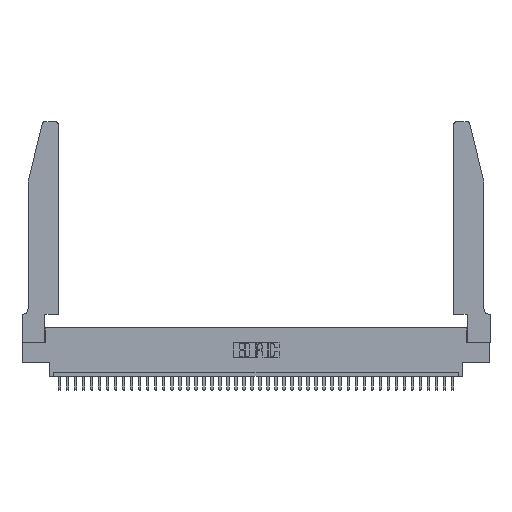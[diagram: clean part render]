
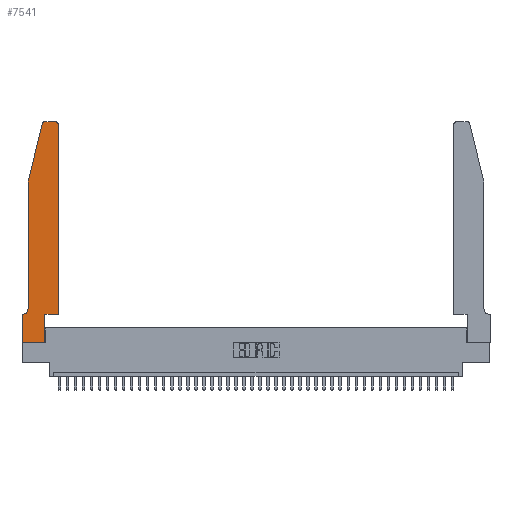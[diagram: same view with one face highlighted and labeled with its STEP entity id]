
A CAD part, top view. The second image highlights one B-rep face of the part: STEP entity #7541.
In plain terms, the highlighted planar face has unit normal (0, 0, 1).
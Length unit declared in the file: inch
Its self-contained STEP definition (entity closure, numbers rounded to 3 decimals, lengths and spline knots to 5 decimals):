
#401 = AXIS2_PLACEMENT_3D ( 'NONE', #15119, #18354, #15260 ) ;
#533 = DIRECTION ( 'NONE',  ( -1., 0., 0. ) ) ;
#1159 = CARTESIAN_POINT ( 'NONE',  ( 0.25487, 2.72718, 0.37 ) ) ;
#1420 = DIRECTION ( 'NONE',  ( 0., -1., 0. ) ) ;
#1784 = ORIENTED_EDGE ( 'NONE', *, *, #6266, .T. ) ;
#2043 = CIRCLE ( 'NONE', #19523, 0.07 ) ;
#2073 = VERTEX_POINT ( 'NONE', #18774 ) ;
#3049 = DIRECTION ( 'NONE',  ( 1., 0., 0. ) ) ;
#3473 = CARTESIAN_POINT ( 'NONE',  ( 0.2865, 0.35, 0.37 ) ) ;
#3515 = VECTOR ( 'NONE', #37276, 39.37008 ) ;
#3591 = VERTEX_POINT ( 'NONE', #35579 ) ;
#3637 = CARTESIAN_POINT ( 'NONE',  ( 0.0055, 0.42, 0.37 ) ) ;
#4028 = CARTESIAN_POINT ( 'NONE',  ( 0.2865, 0.35, 0.37 ) ) ;
#4441 = EDGE_CURVE ( 'NONE', #37183, #3591, #35632, .T. ) ;
#4899 = CARTESIAN_POINT ( 'NONE',  ( 0.0755, 2., 0.37 ) ) ;
#5159 = LINE ( 'NONE', #3473, #18180 ) ;
#5288 = EDGE_LOOP ( 'NONE', ( #20332, #1784, #21687, #19204, #33702, #22159, #9049, #8643, #10576, #39153, #11915, #27888 ) ) ;
#5338 = CARTESIAN_POINT ( 'NONE',  ( 0., 0., 0.37 ) ) ;
#6016 = LINE ( 'NONE', #4899, #24001 ) ;
#6049 = CARTESIAN_POINT ( 'NONE',  ( 0.4505, 0.35, 0.37 ) ) ;
#6266 = EDGE_CURVE ( 'NONE', #37023, #22501, #35423, .T. ) ;
#7541 = ADVANCED_FACE ( 'NONE', ( #9280 ), #37585, .T. ) ;
#8643 = ORIENTED_EDGE ( 'NONE', *, *, #20083, .T. ) ;
#8774 = CARTESIAN_POINT ( 'NONE',  ( 0.0755, 2., 0.37 ) ) ;
#8899 = EDGE_CURVE ( 'NONE', #2073, #14318, #40217, .T. ) ;
#9049 = ORIENTED_EDGE ( 'NONE', *, *, #13860, .T. ) ;
#9280 = FACE_OUTER_BOUND ( 'NONE', #5288, .T. ) ;
#9342 = VERTEX_POINT ( 'NONE', #12655 ) ;
#9844 = CARTESIAN_POINT ( 'NONE',  ( 0.4505, 0.35, 0.37 ) ) ;
#10376 = CARTESIAN_POINT ( 'NONE',  ( 0., 0., 0.37 ) ) ;
#10576 = ORIENTED_EDGE ( 'NONE', *, *, #27069, .T. ) ;
#11915 = ORIENTED_EDGE ( 'NONE', *, *, #14470, .T. ) ;
#12655 = CARTESIAN_POINT ( 'NONE',  ( 0.2865, 0., 0.37 ) ) ;
#13429 = VERTEX_POINT ( 'NONE', #4028 ) ;
#13557 = VECTOR ( 'NONE', #21841, 39.37008 ) ;
#13860 = EDGE_CURVE ( 'NONE', #3591, #31675, #24715, .T. ) ;
#14318 = VERTEX_POINT ( 'NONE', #27202 ) ;
#14462 = VERTEX_POINT ( 'NONE', #39536 ) ;
#14470 = EDGE_CURVE ( 'NONE', #28047, #2073, #21204, .T. ) ;
#15119 = CARTESIAN_POINT ( 'NONE',  ( 0., 0.35, 0.37 ) ) ;
#15260 = DIRECTION ( 'NONE',  ( 1., 0., 0. ) ) ;
#16676 = DIRECTION ( 'NONE',  ( 0., -1., 0. ) ) ;
#17456 = CARTESIAN_POINT ( 'NONE',  ( 0.284, 2.75, 0.37 ) ) ;
#17511 = LINE ( 'NONE', #5338, #38616 ) ;
#18053 = EDGE_CURVE ( 'NONE', #13429, #28047, #31676, .T. ) ;
#18180 = VECTOR ( 'NONE', #38701, 39.37008 ) ;
#18354 = DIRECTION ( 'NONE',  ( 0., 0., 1. ) ) ;
#18675 = DIRECTION ( 'NONE',  ( 0., 0., 1. ) ) ;
#18774 = CARTESIAN_POINT ( 'NONE',  ( 0.4505, 2.72, 0.37 ) ) ;
#19204 = ORIENTED_EDGE ( 'NONE', *, *, #25355, .T. ) ;
#19523 = AXIS2_PLACEMENT_3D ( 'NONE', #3637, #38995, #533 ) ;
#19969 = EDGE_CURVE ( 'NONE', #22501, #31465, #6016, .T. ) ;
#20083 = EDGE_CURVE ( 'NONE', #31675, #9342, #17511, .T. ) ;
#20332 = ORIENTED_EDGE ( 'NONE', *, *, #39080, .T. ) ;
#20580 = DIRECTION ( 'NONE',  ( 0., 1., 0. ) ) ;
#20818 = LINE ( 'NONE', #35754, #21833 ) ;
#20855 = DIRECTION ( 'NONE',  ( 0., 0., 1. ) ) ;
#20931 = CARTESIAN_POINT ( 'NONE',  ( 0., 0., 0.37 ) ) ;
#21123 = CARTESIAN_POINT ( 'NONE',  ( 0.0755, 0.35, 0.37 ) ) ;
#21204 = LINE ( 'NONE', #33334, #21696 ) ;
#21687 = ORIENTED_EDGE ( 'NONE', *, *, #19969, .T. ) ;
#21696 = VECTOR ( 'NONE', #20580, 39.37008 ) ;
#21833 = VECTOR ( 'NONE', #16676, 39.37008 ) ;
#21841 = DIRECTION ( 'NONE',  ( 1., 0., 0. ) ) ;
#22159 = ORIENTED_EDGE ( 'NONE', *, *, #4441, .T. ) ;
#22501 = VERTEX_POINT ( 'NONE', #1159 ) ;
#22619 = CARTESIAN_POINT ( 'NONE',  ( 0.284, 2.72, 0.37 ) ) ;
#24001 = VECTOR ( 'NONE', #27756, 39.37008 ) ;
#24715 = LINE ( 'NONE', #20931, #37827 ) ;
#25355 = EDGE_CURVE ( 'NONE', #31465, #14462, #20818, .T. ) ;
#26736 = VECTOR ( 'NONE', #29137, 39.37008 ) ;
#27069 = EDGE_CURVE ( 'NONE', #9342, #13429, #5159, .T. ) ;
#27202 = CARTESIAN_POINT ( 'NONE',  ( 0.4205, 2.75, 0.37 ) ) ;
#27505 = AXIS2_PLACEMENT_3D ( 'NONE', #22619, #20855, #3049 ) ;
#27756 = DIRECTION ( 'NONE',  ( -0.239, -0.971, 0. ) ) ;
#27888 = ORIENTED_EDGE ( 'NONE', *, *, #8899, .T. ) ;
#28000 = EDGE_CURVE ( 'NONE', #14462, #37183, #2043, .T. ) ;
#28047 = VERTEX_POINT ( 'NONE', #6049 ) ;
#29137 = DIRECTION ( 'NONE',  ( -1., 0., 0. ) ) ;
#29555 = CARTESIAN_POINT ( 'NONE',  ( 0.2605, 2.75, 0.37 ) ) ;
#31465 = VERTEX_POINT ( 'NONE', #8774 ) ;
#31675 = VERTEX_POINT ( 'NONE', #10376 ) ;
#31676 = LINE ( 'NONE', #9844, #13557 ) ;
#31823 = DIRECTION ( 'NONE',  ( 1., 0., 0. ) ) ;
#33334 = CARTESIAN_POINT ( 'NONE',  ( 0.4505, 0.35, 0.37 ) ) ;
#33702 = ORIENTED_EDGE ( 'NONE', *, *, #28000, .T. ) ;
#35423 = CIRCLE ( 'NONE', #27505, 0.03 ) ;
#35579 = CARTESIAN_POINT ( 'NONE',  ( 0., 0.35, 0.37 ) ) ;
#35632 = LINE ( 'NONE', #21123, #3515 ) ;
#35754 = CARTESIAN_POINT ( 'NONE',  ( 0.0755, 2., 0.37 ) ) ;
#37023 = VERTEX_POINT ( 'NONE', #17456 ) ;
#37183 = VERTEX_POINT ( 'NONE', #40647 ) ;
#37276 = DIRECTION ( 'NONE',  ( -1., 0., 0. ) ) ;
#37310 = DIRECTION ( 'NONE',  ( 1., 0., 0. ) ) ;
#37333 = LINE ( 'NONE', #29555, #26736 ) ;
#37585 = PLANE ( 'NONE',  #401 ) ;
#37827 = VECTOR ( 'NONE', #1420, 39.37008 ) ;
#38616 = VECTOR ( 'NONE', #37310, 39.37008 ) ;
#38701 = DIRECTION ( 'NONE',  ( 0., 1., 0. ) ) ;
#38995 = DIRECTION ( 'NONE',  ( 0., 0., -1. ) ) ;
#39080 = EDGE_CURVE ( 'NONE', #14318, #37023, #37333, .T. ) ;
#39153 = ORIENTED_EDGE ( 'NONE', *, *, #18053, .T. ) ;
#39536 = CARTESIAN_POINT ( 'NONE',  ( 0.0755, 0.42, 0.37 ) ) ;
#39681 = AXIS2_PLACEMENT_3D ( 'NONE', #41009, #18675, #31823 ) ;
#40217 = CIRCLE ( 'NONE', #39681, 0.03 ) ;
#40647 = CARTESIAN_POINT ( 'NONE',  ( 0.0055, 0.35, 0.37 ) ) ;
#41009 = CARTESIAN_POINT ( 'NONE',  ( 0.4205, 2.72, 0.37 ) ) ;
